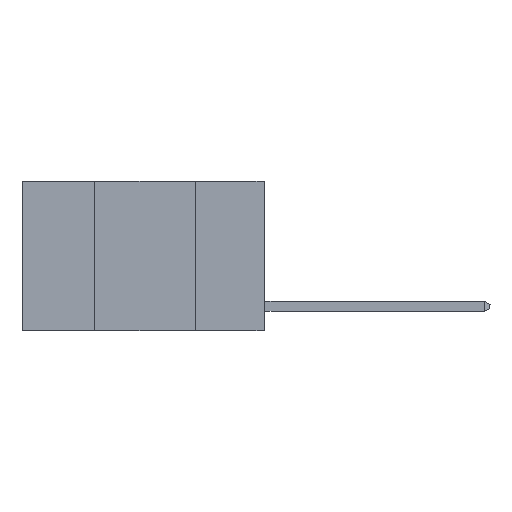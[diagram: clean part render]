
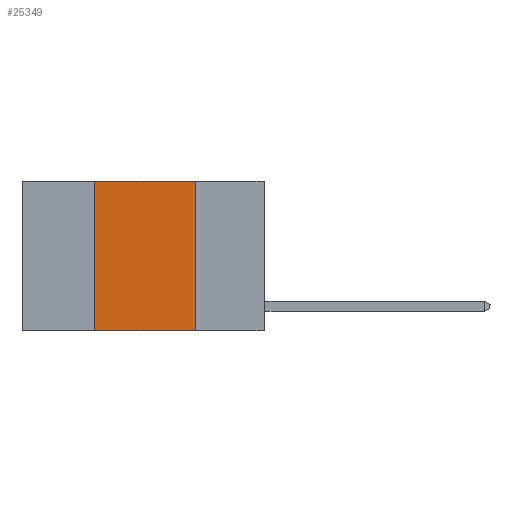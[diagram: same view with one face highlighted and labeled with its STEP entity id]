
A CAD part, left-side view. The second image highlights one B-rep face of the part: STEP entity #25349.
In plain terms, the highlighted planar face has unit normal (-1, 0, 0).
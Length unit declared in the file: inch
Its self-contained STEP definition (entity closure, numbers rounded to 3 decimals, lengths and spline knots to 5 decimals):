
#5 = CARTESIAN_POINT ( 'NONE',  ( 0., 0.17, -0.37 ) ) ;
#390 = EDGE_CURVE ( 'NONE', #26034, #17341, #16871, .T. ) ;
#912 = LINE ( 'NONE', #10304, #6021 ) ;
#1236 = DIRECTION ( 'NONE',  ( 0., -1., 0. ) ) ;
#1803 = CARTESIAN_POINT ( 'NONE',  ( 0., 0.42, 0. ) ) ;
#2167 = LINE ( 'NONE', #17827, #3137 ) ;
#3137 = VECTOR ( 'NONE', #1236, 39.37008 ) ;
#3218 = AXIS2_PLACEMENT_3D ( 'NONE', #5256, #7003, #5083 ) ;
#3968 = VECTOR ( 'NONE', #6775, 39.37008 ) ;
#4434 = CARTESIAN_POINT ( 'NONE',  ( 0., 0.42, 0. ) ) ;
#5083 = DIRECTION ( 'NONE',  ( 0., 0., -1. ) ) ;
#5256 = CARTESIAN_POINT ( 'NONE',  ( 0., 0.6, 0. ) ) ;
#5971 = EDGE_LOOP ( 'NONE', ( #20858, #19328, #10565, #22489 ) ) ;
#6021 = VECTOR ( 'NONE', #24640, 39.37008 ) ;
#6775 = DIRECTION ( 'NONE',  ( 0., 0., 1. ) ) ;
#7003 = DIRECTION ( 'NONE',  ( 1., 0., 0. ) ) ;
#7699 = EDGE_CURVE ( 'NONE', #17341, #13664, #912, .T. ) ;
#10304 = CARTESIAN_POINT ( 'NONE',  ( 0., 0.6, 0. ) ) ;
#10436 = CARTESIAN_POINT ( 'NONE',  ( 0., 0.17, 0. ) ) ;
#10565 = ORIENTED_EDGE ( 'NONE', *, *, #390, .F. ) ;
#11617 = VECTOR ( 'NONE', #20150, 39.37008 ) ;
#12594 = LINE ( 'NONE', #24132, #11617 ) ;
#13664 = VERTEX_POINT ( 'NONE', #10436 ) ;
#16871 = LINE ( 'NONE', #4434, #3968 ) ;
#17341 = VERTEX_POINT ( 'NONE', #1803 ) ;
#17827 = CARTESIAN_POINT ( 'NONE',  ( 0., 0.6, -0.37 ) ) ;
#19028 = EDGE_CURVE ( 'NONE', #13664, #25156, #12594, .T. ) ;
#19328 = ORIENTED_EDGE ( 'NONE', *, *, #7699, .F. ) ;
#19393 = PLANE ( 'NONE',  #3218 ) ;
#19713 = FACE_OUTER_BOUND ( 'NONE', #5971, .T. ) ;
#20150 = DIRECTION ( 'NONE',  ( 0., 0., -1. ) ) ;
#20858 = ORIENTED_EDGE ( 'NONE', *, *, #19028, .F. ) ;
#22489 = ORIENTED_EDGE ( 'NONE', *, *, #26674, .T. ) ;
#23764 = CARTESIAN_POINT ( 'NONE',  ( 0., 0.42, -0.37 ) ) ;
#24132 = CARTESIAN_POINT ( 'NONE',  ( 0., 0.17, 0. ) ) ;
#24640 = DIRECTION ( 'NONE',  ( 0., -1., 0. ) ) ;
#25156 = VERTEX_POINT ( 'NONE', #5 ) ;
#25349 = ADVANCED_FACE ( 'NONE', ( #19713 ), #19393, .F. ) ;
#26034 = VERTEX_POINT ( 'NONE', #23764 ) ;
#26674 = EDGE_CURVE ( 'NONE', #26034, #25156, #2167, .T. ) ;
